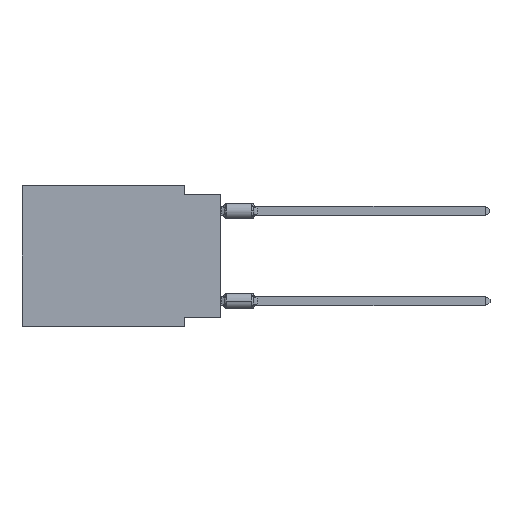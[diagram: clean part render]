
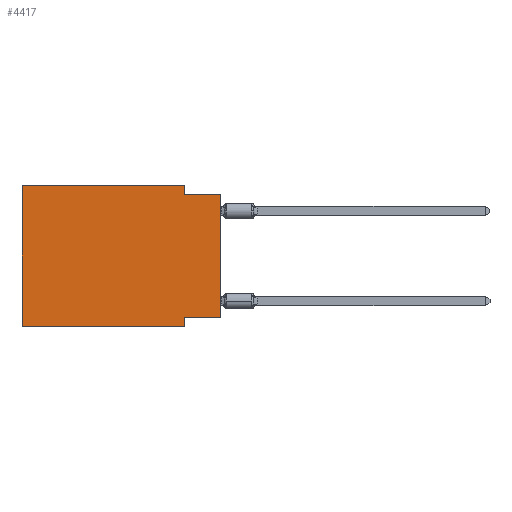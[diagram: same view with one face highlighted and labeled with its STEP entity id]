
A CAD part, left-side view. The second image highlights one B-rep face of the part: STEP entity #4417.
In plain terms, the highlighted planar face has unit normal (-1, 0, 0).
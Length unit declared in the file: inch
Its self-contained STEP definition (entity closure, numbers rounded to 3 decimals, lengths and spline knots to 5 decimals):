
#459 = DIRECTION ( 'NONE',  ( 1., 0., 0. ) ) ;
#505 = VECTOR ( 'NONE', #7343, 39.37008 ) ;
#909 = EDGE_CURVE ( 'NONE', #12693, #4689, #16869, .T. ) ;
#1355 = CARTESIAN_POINT ( 'NONE',  ( 0., 0.1, -0.365 ) ) ;
#1589 = ORIENTED_EDGE ( 'NONE', *, *, #909, .T. ) ;
#1899 = LINE ( 'NONE', #3744, #17114 ) ;
#2085 = VECTOR ( 'NONE', #20484, 39.37008 ) ;
#2271 = EDGE_CURVE ( 'NONE', #7946, #13576, #1899, .T. ) ;
#2533 = EDGE_CURVE ( 'NONE', #14002, #10718, #20542, .T. ) ;
#3593 = VECTOR ( 'NONE', #20329, 39.37008 ) ;
#3662 = CARTESIAN_POINT ( 'NONE',  ( 0., 0.1, -0.39 ) ) ;
#3706 = LINE ( 'NONE', #12222, #5117 ) ;
#3744 = CARTESIAN_POINT ( 'NONE',  ( 0., 0., -0.365 ) ) ;
#4143 = CARTESIAN_POINT ( 'NONE',  ( 0., 0.55, 0. ) ) ;
#4306 = ORIENTED_EDGE ( 'NONE', *, *, #17220, .F. ) ;
#4396 = EDGE_CURVE ( 'NONE', #14750, #11835, #19926, .T. ) ;
#4417 = ADVANCED_FACE ( 'NONE', ( #14505 ), #9224, .F. ) ;
#4689 = VERTEX_POINT ( 'NONE', #21296 ) ;
#4768 = DIRECTION ( 'NONE',  ( 0., -1., 0. ) ) ;
#4818 = CARTESIAN_POINT ( 'NONE',  ( 0., 0., -0.025 ) ) ;
#5117 = VECTOR ( 'NONE', #9001, 39.37008 ) ;
#5214 = VECTOR ( 'NONE', #11164, 39.37008 ) ;
#6434 = CARTESIAN_POINT ( 'NONE',  ( 0., 0.1, 0. ) ) ;
#7343 = DIRECTION ( 'NONE',  ( 0., 0., -1. ) ) ;
#7946 = VERTEX_POINT ( 'NONE', #9468 ) ;
#9001 = DIRECTION ( 'NONE',  ( 0., 0., 1. ) ) ;
#9224 = PLANE ( 'NONE',  #11079 ) ;
#9468 = CARTESIAN_POINT ( 'NONE',  ( 0., 0., -0.365 ) ) ;
#9836 = EDGE_CURVE ( 'NONE', #13576, #4689, #12630, .T. ) ;
#10135 = VECTOR ( 'NONE', #18447, 39.37008 ) ;
#10179 = CARTESIAN_POINT ( 'NONE',  ( 0., 0., -0.025 ) ) ;
#10718 = VERTEX_POINT ( 'NONE', #4818 ) ;
#11079 = AXIS2_PLACEMENT_3D ( 'NONE', #16344, #459, #21777 ) ;
#11164 = DIRECTION ( 'NONE',  ( 0., -1., 0. ) ) ;
#11402 = CARTESIAN_POINT ( 'NONE',  ( 0., 0., 0. ) ) ;
#11835 = VERTEX_POINT ( 'NONE', #6434 ) ;
#12222 = CARTESIAN_POINT ( 'NONE',  ( 0., 0.55, 0. ) ) ;
#12262 = DIRECTION ( 'NONE',  ( 0., 1., 0. ) ) ;
#12630 = LINE ( 'NONE', #3662, #505 ) ;
#12693 = VERTEX_POINT ( 'NONE', #22725 ) ;
#13022 = EDGE_CURVE ( 'NONE', #7946, #10718, #18088, .T. ) ;
#13121 = EDGE_LOOP ( 'NONE', ( #18519, #16971, #19938, #13538, #4306, #1589, #16426, #15346 ) ) ;
#13463 = LINE ( 'NONE', #18986, #2085 ) ;
#13538 = ORIENTED_EDGE ( 'NONE', *, *, #4396, .F. ) ;
#13576 = VERTEX_POINT ( 'NONE', #1355 ) ;
#14002 = VERTEX_POINT ( 'NONE', #19273 ) ;
#14505 = FACE_OUTER_BOUND ( 'NONE', #13121, .T. ) ;
#14750 = VERTEX_POINT ( 'NONE', #18995 ) ;
#15346 = ORIENTED_EDGE ( 'NONE', *, *, #2271, .F. ) ;
#16344 = CARTESIAN_POINT ( 'NONE',  ( 0., 0.55, 0. ) ) ;
#16426 = ORIENTED_EDGE ( 'NONE', *, *, #9836, .F. ) ;
#16869 = LINE ( 'NONE', #19869, #3593 ) ;
#16971 = ORIENTED_EDGE ( 'NONE', *, *, #2533, .F. ) ;
#17114 = VECTOR ( 'NONE', #12262, 39.37008 ) ;
#17220 = EDGE_CURVE ( 'NONE', #12693, #14750, #3706, .T. ) ;
#18088 = LINE ( 'NONE', #11402, #10135 ) ;
#18131 = EDGE_CURVE ( 'NONE', #11835, #14002, #13463, .T. ) ;
#18447 = DIRECTION ( 'NONE',  ( 0., 0., 1. ) ) ;
#18519 = ORIENTED_EDGE ( 'NONE', *, *, #13022, .T. ) ;
#18750 = VECTOR ( 'NONE', #4768, 39.37008 ) ;
#18986 = CARTESIAN_POINT ( 'NONE',  ( 0., 0.1, 0. ) ) ;
#18995 = CARTESIAN_POINT ( 'NONE',  ( 0., 0.55, 0. ) ) ;
#19273 = CARTESIAN_POINT ( 'NONE',  ( 0., 0.1, -0.025 ) ) ;
#19869 = CARTESIAN_POINT ( 'NONE',  ( 0., 0.55, -0.39 ) ) ;
#19926 = LINE ( 'NONE', #4143, #5214 ) ;
#19938 = ORIENTED_EDGE ( 'NONE', *, *, #18131, .F. ) ;
#20329 = DIRECTION ( 'NONE',  ( 0., -1., 0. ) ) ;
#20484 = DIRECTION ( 'NONE',  ( 0., 0., -1. ) ) ;
#20542 = LINE ( 'NONE', #10179, #18750 ) ;
#21296 = CARTESIAN_POINT ( 'NONE',  ( 0., 0.1, -0.39 ) ) ;
#21777 = DIRECTION ( 'NONE',  ( 0., 0., -1. ) ) ;
#22725 = CARTESIAN_POINT ( 'NONE',  ( 0., 0.55, -0.39 ) ) ;
